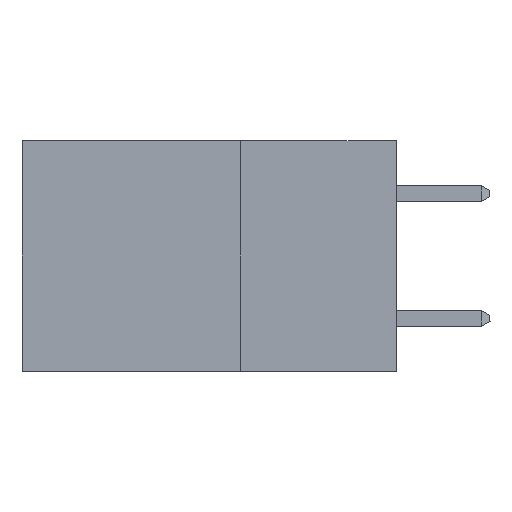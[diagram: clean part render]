
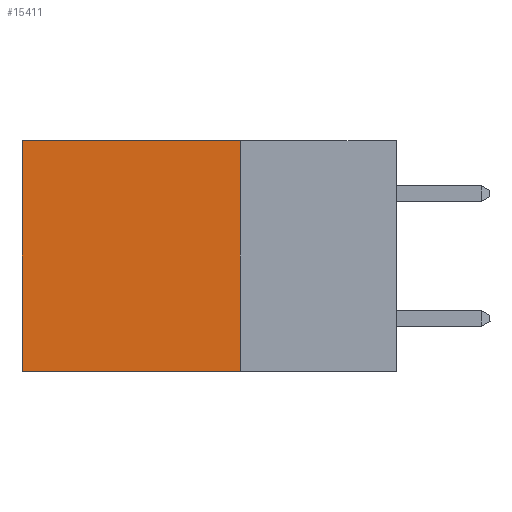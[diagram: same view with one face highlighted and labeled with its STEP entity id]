
A CAD part, left-side view. The second image highlights one B-rep face of the part: STEP entity #15411.
In plain terms, the highlighted planar face has unit normal (-1, 0, 0).
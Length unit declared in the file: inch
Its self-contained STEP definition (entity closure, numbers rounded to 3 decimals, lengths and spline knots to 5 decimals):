
#722 = VECTOR ( 'NONE', #22913, 39.37008 ) ;
#1274 = VERTEX_POINT ( 'NONE', #21329 ) ;
#1440 = VERTEX_POINT ( 'NONE', #19647 ) ;
#1694 = VECTOR ( 'NONE', #10822, 39.37008 ) ;
#3245 = VERTEX_POINT ( 'NONE', #23423 ) ;
#3489 = PLANE ( 'NONE',  #13864 ) ;
#3744 = CARTESIAN_POINT ( 'NONE',  ( 0.298, 0.25, 0. ) ) ;
#4668 = LINE ( 'NONE', #19049, #19384 ) ;
#5770 = DIRECTION ( 'NONE',  ( 0., 0., -1. ) ) ;
#6522 = CARTESIAN_POINT ( 'NONE',  ( 0.298, 0.25, 0. ) ) ;
#6617 = VERTEX_POINT ( 'NONE', #8730 ) ;
#8730 = CARTESIAN_POINT ( 'NONE',  ( 0.298, 0.25, -0.37 ) ) ;
#9095 = VECTOR ( 'NONE', #19859, 39.37008 ) ;
#9554 = DIRECTION ( 'NONE',  ( 0., 0., -1. ) ) ;
#10822 = DIRECTION ( 'NONE',  ( 0., 0., -1. ) ) ;
#12385 = ORIENTED_EDGE ( 'NONE', *, *, #22222, .T. ) ;
#13864 = AXIS2_PLACEMENT_3D ( 'NONE', #3744, #17259, #5770 ) ;
#14751 = LINE ( 'NONE', #6522, #9095 ) ;
#15411 = ADVANCED_FACE ( 'NONE', ( #18800 ), #3489, .F. ) ;
#15800 = ORIENTED_EDGE ( 'NONE', *, *, #19183, .T. ) ;
#16195 = LINE ( 'NONE', #19138, #722 ) ;
#17259 = DIRECTION ( 'NONE',  ( 1., 0., 0. ) ) ;
#18541 = ORIENTED_EDGE ( 'NONE', *, *, #19415, .F. ) ;
#18800 = FACE_OUTER_BOUND ( 'NONE', #20341, .T. ) ;
#19049 = CARTESIAN_POINT ( 'NONE',  ( 0.298, 0.25, 0. ) ) ;
#19138 = CARTESIAN_POINT ( 'NONE',  ( 0.298, 0.25, -0.37 ) ) ;
#19183 = EDGE_CURVE ( 'NONE', #1274, #1440, #22147, .T. ) ;
#19384 = VECTOR ( 'NONE', #9554, 39.37008 ) ;
#19415 = EDGE_CURVE ( 'NONE', #6617, #1440, #16195, .T. ) ;
#19647 = CARTESIAN_POINT ( 'NONE',  ( 0.298, 0.6, -0.37 ) ) ;
#19859 = DIRECTION ( 'NONE',  ( 0., 1., 0. ) ) ;
#20121 = ORIENTED_EDGE ( 'NONE', *, *, #24481, .F. ) ;
#20281 = CARTESIAN_POINT ( 'NONE',  ( 0.298, 0.6, 0. ) ) ;
#20341 = EDGE_LOOP ( 'NONE', ( #15800, #18541, #20121, #12385 ) ) ;
#21329 = CARTESIAN_POINT ( 'NONE',  ( 0.298, 0.6, 0. ) ) ;
#22147 = LINE ( 'NONE', #20281, #1694 ) ;
#22222 = EDGE_CURVE ( 'NONE', #3245, #1274, #14751, .T. ) ;
#22913 = DIRECTION ( 'NONE',  ( 0., 1., 0. ) ) ;
#23423 = CARTESIAN_POINT ( 'NONE',  ( 0.298, 0.25, 0. ) ) ;
#24481 = EDGE_CURVE ( 'NONE', #3245, #6617, #4668, .T. ) ;
